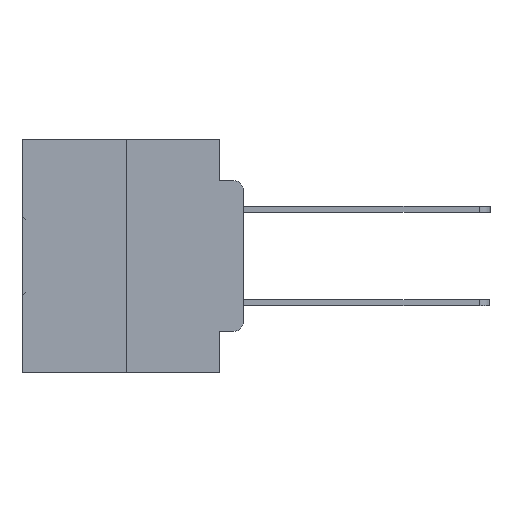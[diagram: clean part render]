
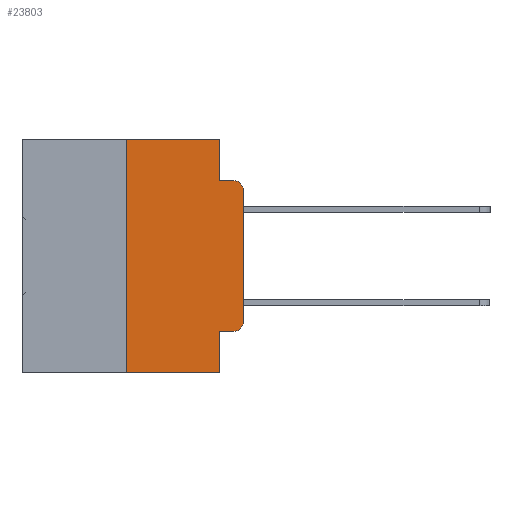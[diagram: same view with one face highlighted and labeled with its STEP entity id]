
A CAD part, left-side view. The second image highlights one B-rep face of the part: STEP entity #23803.
In plain terms, the highlighted planar face has unit normal (-1, 0, 0).
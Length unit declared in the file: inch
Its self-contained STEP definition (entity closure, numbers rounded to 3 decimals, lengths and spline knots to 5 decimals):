
#183 = EDGE_CURVE ( 'NONE', #8695, #29186, #32900, .T. ) ;
#236 = CARTESIAN_POINT ( 'NONE',  ( 0., 0.25, 0. ) ) ;
#386 = CARTESIAN_POINT ( 'NONE',  ( 0., 0.051, 0. ) ) ;
#1138 = VECTOR ( 'NONE', #16054, 39.37008 ) ;
#1518 = VERTEX_POINT ( 'NONE', #21870 ) ;
#1785 = CARTESIAN_POINT ( 'NONE',  ( 0., 0.051, -0.4115 ) ) ;
#2223 = AXIS2_PLACEMENT_3D ( 'NONE', #22110, #6281, #24786 ) ;
#2458 = CARTESIAN_POINT ( 'NONE',  ( 0., 0., 0. ) ) ;
#2714 = EDGE_CURVE ( 'NONE', #8716, #30531, #16872, .T. ) ;
#2905 = DIRECTION ( 'NONE',  ( 0., 0., 1. ) ) ;
#3344 = PLANE ( 'NONE',  #14417 ) ;
#3399 = ORIENTED_EDGE ( 'NONE', *, *, #33169, .T. ) ;
#4050 = AXIS2_PLACEMENT_3D ( 'NONE', #21087, #5273, #23761 ) ;
#4502 = VECTOR ( 'NONE', #2905, 39.37008 ) ;
#4668 = VECTOR ( 'NONE', #30440, 39.37008 ) ;
#5013 = CARTESIAN_POINT ( 'NONE',  ( 0., 0., -0.3915 ) ) ;
#5273 = DIRECTION ( 'NONE',  ( -1., 0., 0. ) ) ;
#5383 = EDGE_CURVE ( 'NONE', #19496, #1518, #17041, .T. ) ;
#6256 = LINE ( 'NONE', #2458, #12455 ) ;
#6281 = DIRECTION ( 'NONE',  ( -1., 0., 0. ) ) ;
#6556 = CARTESIAN_POINT ( 'NONE',  ( 0., 0., -0.1085 ) ) ;
#7537 = EDGE_CURVE ( 'NONE', #19496, #30531, #10447, .T. ) ;
#8695 = VERTEX_POINT ( 'NONE', #27560 ) ;
#8716 = VERTEX_POINT ( 'NONE', #9198 ) ;
#8874 = ORIENTED_EDGE ( 'NONE', *, *, #15073, .T. ) ;
#9065 = CARTESIAN_POINT ( 'NONE',  ( 0., 0.473, 0. ) ) ;
#9198 = CARTESIAN_POINT ( 'NONE',  ( 0., 0.25, -0.5 ) ) ;
#9632 = DIRECTION ( 'NONE',  ( 0., 0., -1. ) ) ;
#10068 = VECTOR ( 'NONE', #21993, 39.37008 ) ;
#10074 = ORIENTED_EDGE ( 'NONE', *, *, #13938, .F. ) ;
#10237 = EDGE_CURVE ( 'NONE', #10972, #28671, #18896, .T. ) ;
#10447 = LINE ( 'NONE', #25543, #30727 ) ;
#10866 = CARTESIAN_POINT ( 'NONE',  ( 0., 0.051, -0.0885 ) ) ;
#10972 = VERTEX_POINT ( 'NONE', #14864 ) ;
#11082 = VECTOR ( 'NONE', #16976, 39.37008 ) ;
#11238 = FACE_OUTER_BOUND ( 'NONE', #30752, .T. ) ;
#11353 = DIRECTION ( 'NONE',  ( 0., 0., -1. ) ) ;
#11849 = CARTESIAN_POINT ( 'NONE',  ( 0., 0.051, -0.5 ) ) ;
#12019 = CIRCLE ( 'NONE', #4050, 0.02 ) ;
#12455 = VECTOR ( 'NONE', #20957, 39.37008 ) ;
#13938 = EDGE_CURVE ( 'NONE', #28671, #8695, #25764, .T. ) ;
#14417 = AXIS2_PLACEMENT_3D ( 'NONE', #29740, #27192, #11353 ) ;
#14519 = VERTEX_POINT ( 'NONE', #6556 ) ;
#14790 = EDGE_CURVE ( 'NONE', #29159, #14519, #6256, .T. ) ;
#14864 = CARTESIAN_POINT ( 'NONE',  ( 0., 0.25, 0. ) ) ;
#14995 = ORIENTED_EDGE ( 'NONE', *, *, #10237, .F. ) ;
#15073 = EDGE_CURVE ( 'NONE', #1518, #29159, #33117, .T. ) ;
#15616 = CARTESIAN_POINT ( 'NONE',  ( 0., 0.473, -0.5 ) ) ;
#16054 = DIRECTION ( 'NONE',  ( 0., -1., 0. ) ) ;
#16872 = LINE ( 'NONE', #15616, #1138 ) ;
#16976 = DIRECTION ( 'NONE',  ( 0., -1., 0. ) ) ;
#17041 = LINE ( 'NONE', #29901, #10068 ) ;
#17481 = ORIENTED_EDGE ( 'NONE', *, *, #2714, .T. ) ;
#18268 = ORIENTED_EDGE ( 'NONE', *, *, #183, .F. ) ;
#18544 = LINE ( 'NONE', #236, #4502 ) ;
#18896 = LINE ( 'NONE', #9065, #11082 ) ;
#19151 = ORIENTED_EDGE ( 'NONE', *, *, #5383, .T. ) ;
#19496 = VERTEX_POINT ( 'NONE', #1785 ) ;
#20957 = DIRECTION ( 'NONE',  ( 0., 0., 1. ) ) ;
#21087 = CARTESIAN_POINT ( 'NONE',  ( 0., 0.02, -0.1085 ) ) ;
#21870 = CARTESIAN_POINT ( 'NONE',  ( 0., 0.02, -0.4115 ) ) ;
#21993 = DIRECTION ( 'NONE',  ( 0., -1., 0. ) ) ;
#22110 = CARTESIAN_POINT ( 'NONE',  ( 0., 0.02, -0.3915 ) ) ;
#23670 = ORIENTED_EDGE ( 'NONE', *, *, #14790, .T. ) ;
#23701 = ORIENTED_EDGE ( 'NONE', *, *, #32128, .F. ) ;
#23761 = DIRECTION ( 'NONE',  ( 0., 0., -1. ) ) ;
#23803 = ADVANCED_FACE ( 'NONE', ( #11238 ), #3344, .F. ) ;
#24786 = DIRECTION ( 'NONE',  ( 0., 0., -1. ) ) ;
#25543 = CARTESIAN_POINT ( 'NONE',  ( 0., 0.051, 0. ) ) ;
#25764 = LINE ( 'NONE', #32924, #4668 ) ;
#25886 = VECTOR ( 'NONE', #34132, 39.37008 ) ;
#27192 = DIRECTION ( 'NONE',  ( 1., 0., 0. ) ) ;
#27560 = CARTESIAN_POINT ( 'NONE',  ( 0., 0.051, -0.0885 ) ) ;
#28671 = VERTEX_POINT ( 'NONE', #386 ) ;
#29159 = VERTEX_POINT ( 'NONE', #5013 ) ;
#29186 = VERTEX_POINT ( 'NONE', #34119 ) ;
#29740 = CARTESIAN_POINT ( 'NONE',  ( 0., 0.473, 0. ) ) ;
#29901 = CARTESIAN_POINT ( 'NONE',  ( 0., 0.051, -0.4115 ) ) ;
#30440 = DIRECTION ( 'NONE',  ( 0., 0., -1. ) ) ;
#30531 = VERTEX_POINT ( 'NONE', #11849 ) ;
#30727 = VECTOR ( 'NONE', #9632, 39.37008 ) ;
#30752 = EDGE_LOOP ( 'NONE', ( #23670, #3399, #18268, #10074, #14995, #23701, #17481, #32382, #19151, #8874 ) ) ;
#32128 = EDGE_CURVE ( 'NONE', #8716, #10972, #18544, .T. ) ;
#32382 = ORIENTED_EDGE ( 'NONE', *, *, #7537, .F. ) ;
#32900 = LINE ( 'NONE', #10866, #25886 ) ;
#32924 = CARTESIAN_POINT ( 'NONE',  ( 0., 0.051, 0. ) ) ;
#33117 = CIRCLE ( 'NONE', #2223, 0.02 ) ;
#33169 = EDGE_CURVE ( 'NONE', #14519, #29186, #12019, .T. ) ;
#34119 = CARTESIAN_POINT ( 'NONE',  ( 0., 0.02, -0.0885 ) ) ;
#34132 = DIRECTION ( 'NONE',  ( 0., -1., 0. ) ) ;
